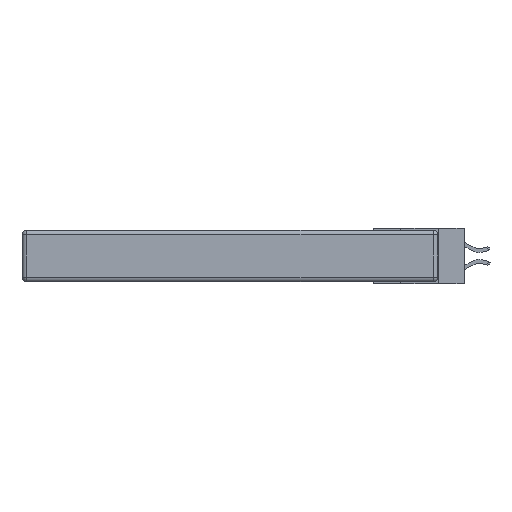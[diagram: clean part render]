
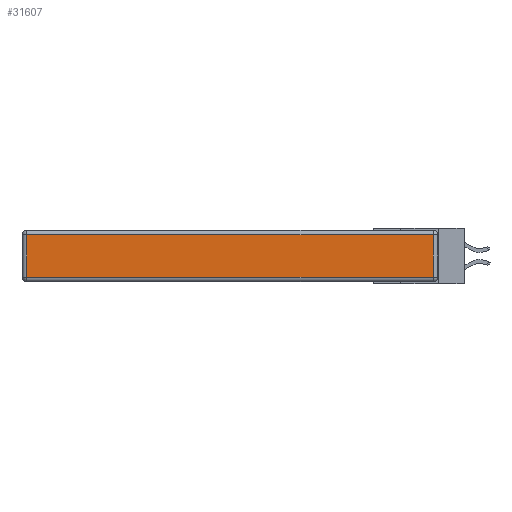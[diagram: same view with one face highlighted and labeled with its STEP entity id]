
A CAD part, left-side view. The second image highlights one B-rep face of the part: STEP entity #31607.
In plain terms, the highlighted planar face has unit normal (-1, 0, 0).
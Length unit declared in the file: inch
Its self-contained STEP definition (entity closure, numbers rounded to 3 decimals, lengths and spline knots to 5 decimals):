
#1254 = VERTEX_POINT ( 'NONE', #25541 ) ;
#2969 = EDGE_CURVE ( 'NONE', #25679, #28710, #17244, .T. ) ;
#3255 = LINE ( 'NONE', #27179, #20508 ) ;
#3567 = ORIENTED_EDGE ( 'NONE', *, *, #2969, .T. ) ;
#3619 = EDGE_CURVE ( 'NONE', #28710, #7404, #28261, .T. ) ;
#6329 = CARTESIAN_POINT ( 'NONE',  ( 0., 2.75, -0.03 ) ) ;
#7209 = EDGE_LOOP ( 'NONE', ( #29478, #16193, #3567, #15109 ) ) ;
#7404 = VERTEX_POINT ( 'NONE', #14532 ) ;
#8012 = VECTOR ( 'NONE', #11273, 39.37008 ) ;
#8793 = EDGE_CURVE ( 'NONE', #1254, #25679, #31193, .T. ) ;
#10518 = DIRECTION ( 'NONE',  ( 0., 0., 1. ) ) ;
#11273 = DIRECTION ( 'NONE',  ( 0., 1., 0. ) ) ;
#11296 = VECTOR ( 'NONE', #31354, 39.37008 ) ;
#13648 = CARTESIAN_POINT ( 'NONE',  ( 0., 2.72, -0.03 ) ) ;
#14532 = CARTESIAN_POINT ( 'NONE',  ( 0., 2.72, -0.313 ) ) ;
#15109 = ORIENTED_EDGE ( 'NONE', *, *, #3619, .T. ) ;
#16193 = ORIENTED_EDGE ( 'NONE', *, *, #8793, .T. ) ;
#16469 = DIRECTION ( 'NONE',  ( 0., 0., 1. ) ) ;
#17244 = LINE ( 'NONE', #6329, #8012 ) ;
#17621 = PLANE ( 'NONE',  #27698 ) ;
#20484 = CARTESIAN_POINT ( 'NONE',  ( 0., 0.03, -0.03 ) ) ;
#20508 = VECTOR ( 'NONE', #31703, 39.37008 ) ;
#22691 = DIRECTION ( 'NONE',  ( -1., 0., 0. ) ) ;
#23604 = CARTESIAN_POINT ( 'NONE',  ( 0., 0.03, -0.343 ) ) ;
#25541 = CARTESIAN_POINT ( 'NONE',  ( 0., 0.03, -0.313 ) ) ;
#25679 = VERTEX_POINT ( 'NONE', #20484 ) ;
#26288 = EDGE_CURVE ( 'NONE', #7404, #1254, #3255, .T. ) ;
#27102 = FACE_OUTER_BOUND ( 'NONE', #7209, .T. ) ;
#27179 = CARTESIAN_POINT ( 'NONE',  ( 0., 0., -0.313 ) ) ;
#27347 = VECTOR ( 'NONE', #16469, 39.37008 ) ;
#27698 = AXIS2_PLACEMENT_3D ( 'NONE', #27737, #22691, #10518 ) ;
#27737 = CARTESIAN_POINT ( 'NONE',  ( 0., 0., -0.343 ) ) ;
#28261 = LINE ( 'NONE', #28600, #11296 ) ;
#28600 = CARTESIAN_POINT ( 'NONE',  ( 0., 2.72, -0.343 ) ) ;
#28710 = VERTEX_POINT ( 'NONE', #13648 ) ;
#29478 = ORIENTED_EDGE ( 'NONE', *, *, #26288, .T. ) ;
#31193 = LINE ( 'NONE', #23604, #27347 ) ;
#31354 = DIRECTION ( 'NONE',  ( 0., 0., -1. ) ) ;
#31607 = ADVANCED_FACE ( 'NONE', ( #27102 ), #17621, .T. ) ;
#31703 = DIRECTION ( 'NONE',  ( 0., -1., 0. ) ) ;
